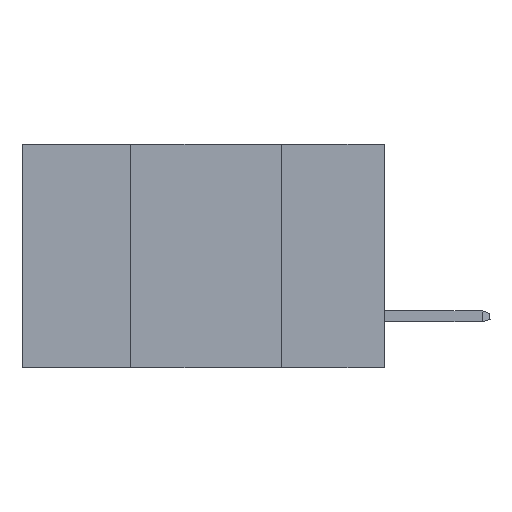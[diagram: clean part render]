
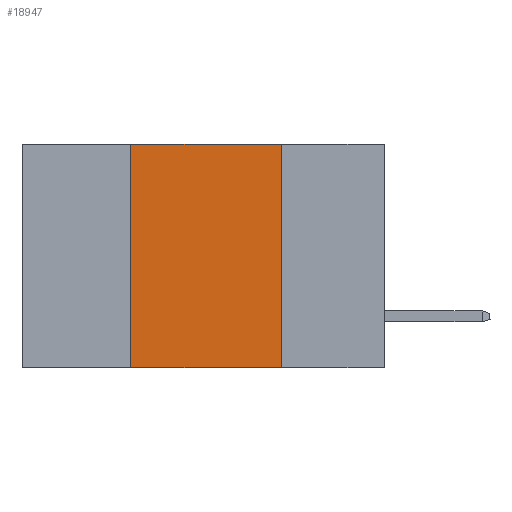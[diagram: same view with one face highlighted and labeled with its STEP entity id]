
A CAD part, left-side view. The second image highlights one B-rep face of the part: STEP entity #18947.
In plain terms, the highlighted planar face has unit normal (-1, 0, 0).
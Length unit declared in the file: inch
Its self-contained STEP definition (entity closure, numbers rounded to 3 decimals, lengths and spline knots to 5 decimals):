
#66 = CARTESIAN_POINT ( 'NONE',  ( 0., 0.17, -0.37 ) ) ;
#204 = VERTEX_POINT ( 'NONE', #66 ) ;
#497 = ORIENTED_EDGE ( 'NONE', *, *, #5251, .F. ) ;
#2536 = VECTOR ( 'NONE', #17682, 39.37008 ) ;
#2574 = VERTEX_POINT ( 'NONE', #12996 ) ;
#3729 = ORIENTED_EDGE ( 'NONE', *, *, #8778, .F. ) ;
#3904 = EDGE_CURVE ( 'NONE', #19867, #204, #22332, .T. ) ;
#5251 = EDGE_CURVE ( 'NONE', #23057, #19867, #8512, .T. ) ;
#5283 = CARTESIAN_POINT ( 'NONE',  ( 0., 0.17, 0. ) ) ;
#5487 = VECTOR ( 'NONE', #23160, 39.37008 ) ;
#6683 = CARTESIAN_POINT ( 'NONE',  ( 0., 0.6, 0. ) ) ;
#6789 = FACE_OUTER_BOUND ( 'NONE', #8169, .T. ) ;
#6928 = LINE ( 'NONE', #18676, #14456 ) ;
#7384 = DIRECTION ( 'NONE',  ( 1., 0., 0. ) ) ;
#7540 = DIRECTION ( 'NONE',  ( 0., 0., -1. ) ) ;
#7782 = EDGE_CURVE ( 'NONE', #2574, #204, #6928, .T. ) ;
#8156 = CARTESIAN_POINT ( 'NONE',  ( 0., 0.17, 0. ) ) ;
#8169 = EDGE_LOOP ( 'NONE', ( #9227, #497, #3729, #12427 ) ) ;
#8512 = LINE ( 'NONE', #6683, #9971 ) ;
#8778 = EDGE_CURVE ( 'NONE', #2574, #23057, #22271, .T. ) ;
#9170 = CARTESIAN_POINT ( 'NONE',  ( 0., 0.6, 0. ) ) ;
#9227 = ORIENTED_EDGE ( 'NONE', *, *, #3904, .F. ) ;
#9971 = VECTOR ( 'NONE', #10246, 39.37008 ) ;
#10210 = CARTESIAN_POINT ( 'NONE',  ( 0., 0.42, 0. ) ) ;
#10246 = DIRECTION ( 'NONE',  ( 0., -1., 0. ) ) ;
#11372 = DIRECTION ( 'NONE',  ( 0., -1., 0. ) ) ;
#12294 = CARTESIAN_POINT ( 'NONE',  ( 0., 0.42, 0. ) ) ;
#12427 = ORIENTED_EDGE ( 'NONE', *, *, #7782, .T. ) ;
#12996 = CARTESIAN_POINT ( 'NONE',  ( 0., 0.42, -0.37 ) ) ;
#13726 = AXIS2_PLACEMENT_3D ( 'NONE', #9170, #7384, #7540 ) ;
#14456 = VECTOR ( 'NONE', #11372, 39.37008 ) ;
#16569 = PLANE ( 'NONE',  #13726 ) ;
#17682 = DIRECTION ( 'NONE',  ( 0., 0., 1. ) ) ;
#18676 = CARTESIAN_POINT ( 'NONE',  ( 0., 0.6, -0.37 ) ) ;
#18947 = ADVANCED_FACE ( 'NONE', ( #6789 ), #16569, .F. ) ;
#19867 = VERTEX_POINT ( 'NONE', #5283 ) ;
#22271 = LINE ( 'NONE', #10210, #2536 ) ;
#22332 = LINE ( 'NONE', #8156, #5487 ) ;
#23057 = VERTEX_POINT ( 'NONE', #12294 ) ;
#23160 = DIRECTION ( 'NONE',  ( 0., 0., -1. ) ) ;
